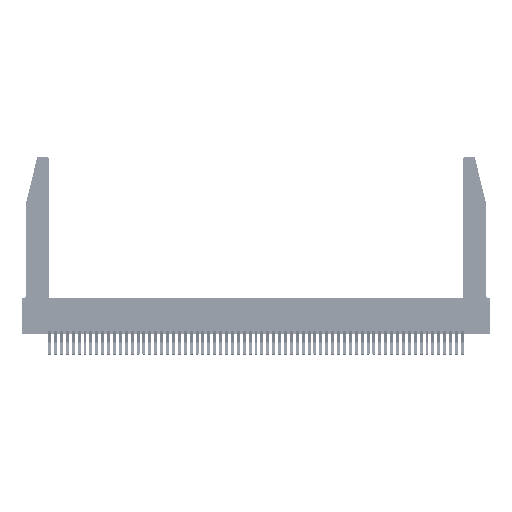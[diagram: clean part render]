
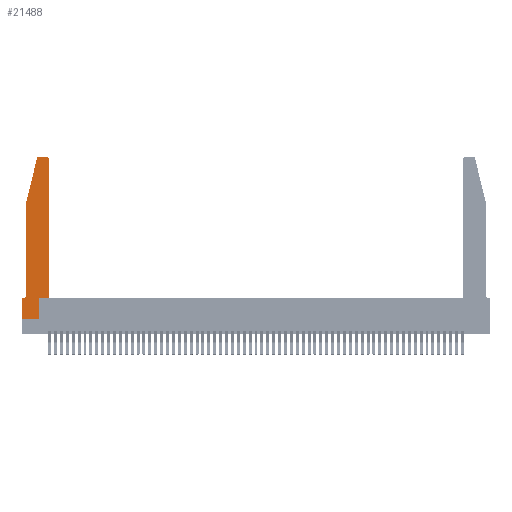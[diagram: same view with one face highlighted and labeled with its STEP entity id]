
A CAD part, top view. The second image highlights one B-rep face of the part: STEP entity #21488.
In plain terms, the highlighted planar face has unit normal (0, 0, 1).
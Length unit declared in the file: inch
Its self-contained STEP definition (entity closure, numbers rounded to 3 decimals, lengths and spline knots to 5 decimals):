
#803 = CARTESIAN_POINT ( 'NONE',  ( 0.0755, 2., 0.37 ) ) ;
#804 = EDGE_CURVE ( 'NONE', #41750, #5095, #30025, .T. ) ;
#1301 = CARTESIAN_POINT ( 'NONE',  ( 0.2865, 0., 0.37 ) ) ;
#1387 = CARTESIAN_POINT ( 'NONE',  ( 0.0055, 0.42, 0.37 ) ) ;
#2762 = VECTOR ( 'NONE', #8914, 39.37008 ) ;
#2973 = VECTOR ( 'NONE', #46245, 39.37008 ) ;
#4022 = EDGE_CURVE ( 'NONE', #11858, #41750, #15976, .T. ) ;
#4548 = VECTOR ( 'NONE', #15993, 39.37008 ) ;
#4670 = CARTESIAN_POINT ( 'NONE',  ( 0.4505, 0.35, 0.37 ) ) ;
#5095 = VERTEX_POINT ( 'NONE', #20547 ) ;
#5931 = DIRECTION ( 'NONE',  ( -1., 0., 0. ) ) ;
#6872 = VERTEX_POINT ( 'NONE', #18686 ) ;
#7213 = AXIS2_PLACEMENT_3D ( 'NONE', #19951, #37444, #11291 ) ;
#8715 = EDGE_LOOP ( 'NONE', ( #17613, #49337, #32407, #40443, #55276, #13586, #16196, #44043, #39970, #46020, #36558, #36023 ) ) ;
#8914 = DIRECTION ( 'NONE',  ( 0., -1., 0. ) ) ;
#9158 = DIRECTION ( 'NONE',  ( 1., 0., 0. ) ) ;
#9674 = LINE ( 'NONE', #45506, #54585 ) ;
#10699 = VERTEX_POINT ( 'NONE', #1301 ) ;
#11068 = VERTEX_POINT ( 'NONE', #38707 ) ;
#11097 = CIRCLE ( 'NONE', #44662, 0.03 ) ;
#11291 = DIRECTION ( 'NONE',  ( 1., 0., 0. ) ) ;
#11606 = EDGE_CURVE ( 'NONE', #55466, #10699, #17693, .T. ) ;
#11858 = VERTEX_POINT ( 'NONE', #48084 ) ;
#13586 = ORIENTED_EDGE ( 'NONE', *, *, #37803, .T. ) ;
#15199 = VECTOR ( 'NONE', #48949, 39.37008 ) ;
#15976 = LINE ( 'NONE', #48135, #2762 ) ;
#15993 = DIRECTION ( 'NONE',  ( 1., 0., 0. ) ) ;
#16196 = ORIENTED_EDGE ( 'NONE', *, *, #45359, .T. ) ;
#16296 = EDGE_CURVE ( 'NONE', #11068, #45266, #41244, .T. ) ;
#16573 = LINE ( 'NONE', #44597, #15199 ) ;
#16674 = CARTESIAN_POINT ( 'NONE',  ( 0.284, 2.72, 0.37 ) ) ;
#16882 = EDGE_CURVE ( 'NONE', #45266, #42300, #21484, .T. ) ;
#17613 = ORIENTED_EDGE ( 'NONE', *, *, #40620, .T. ) ;
#17693 = LINE ( 'NONE', #37718, #4548 ) ;
#17854 = VERTEX_POINT ( 'NONE', #32151 ) ;
#18579 = DIRECTION ( 'NONE',  ( 0., 0., 1. ) ) ;
#18686 = CARTESIAN_POINT ( 'NONE',  ( 0.284, 2.75, 0.37 ) ) ;
#19951 = CARTESIAN_POINT ( 'NONE',  ( 0., 0.35, 0.37 ) ) ;
#20547 = CARTESIAN_POINT ( 'NONE',  ( 0.0055, 0.35, 0.37 ) ) ;
#21099 = DIRECTION ( 'NONE',  ( 1., 0., 0. ) ) ;
#21484 = LINE ( 'NONE', #26206, #54690 ) ;
#21488 = ADVANCED_FACE ( 'NONE', ( #25038 ), #33116, .T. ) ;
#21638 = EDGE_CURVE ( 'NONE', #6872, #38180, #51411, .T. ) ;
#23947 = DIRECTION ( 'NONE',  ( -1., 0., 0. ) ) ;
#24023 = AXIS2_PLACEMENT_3D ( 'NONE', #1387, #32205, #5931 ) ;
#25038 = FACE_OUTER_BOUND ( 'NONE', #8715, .T. ) ;
#26206 = CARTESIAN_POINT ( 'NONE',  ( 0.4505, 0.35, 0.37 ) ) ;
#26783 = EDGE_CURVE ( 'NONE', #42300, #32089, #11097, .T. ) ;
#27752 = CARTESIAN_POINT ( 'NONE',  ( 0.4505, 2.72, 0.37 ) ) ;
#30025 = CIRCLE ( 'NONE', #24023, 0.07 ) ;
#30193 = CARTESIAN_POINT ( 'NONE',  ( 0.4505, 0.35, 0.37 ) ) ;
#30528 = DIRECTION ( 'NONE',  ( 0., 1., 0. ) ) ;
#30736 = AXIS2_PLACEMENT_3D ( 'NONE', #16674, #47074, #21099 ) ;
#31687 = DIRECTION ( 'NONE',  ( -0.239, -0.971, 0. ) ) ;
#32089 = VERTEX_POINT ( 'NONE', #39463 ) ;
#32151 = CARTESIAN_POINT ( 'NONE',  ( 0., 0.35, 0.37 ) ) ;
#32205 = DIRECTION ( 'NONE',  ( 0., 0., -1. ) ) ;
#32407 = ORIENTED_EDGE ( 'NONE', *, *, #42844, .T. ) ;
#33116 = PLANE ( 'NONE',  #7213 ) ;
#33411 = CARTESIAN_POINT ( 'NONE',  ( 0.2605, 2.75, 0.37 ) ) ;
#35023 = LINE ( 'NONE', #803, #45172 ) ;
#35095 = CARTESIAN_POINT ( 'NONE',  ( 0.25487, 2.72718, 0.37 ) ) ;
#36023 = ORIENTED_EDGE ( 'NONE', *, *, #26783, .T. ) ;
#36558 = ORIENTED_EDGE ( 'NONE', *, *, #16882, .T. ) ;
#36648 = LINE ( 'NONE', #33411, #2973 ) ;
#37444 = DIRECTION ( 'NONE',  ( 0., 0., 1. ) ) ;
#37659 = EDGE_CURVE ( 'NONE', #10699, #11068, #16573, .T. ) ;
#37718 = CARTESIAN_POINT ( 'NONE',  ( 0., 0., 0.37 ) ) ;
#37803 = EDGE_CURVE ( 'NONE', #5095, #17854, #9674, .T. ) ;
#38180 = VERTEX_POINT ( 'NONE', #35095 ) ;
#38308 = CARTESIAN_POINT ( 'NONE',  ( 0., 0., 0.37 ) ) ;
#38707 = CARTESIAN_POINT ( 'NONE',  ( 0.2865, 0.35, 0.37 ) ) ;
#39460 = CARTESIAN_POINT ( 'NONE',  ( 0., 0., 0.37 ) ) ;
#39463 = CARTESIAN_POINT ( 'NONE',  ( 0.4205, 2.75, 0.37 ) ) ;
#39970 = ORIENTED_EDGE ( 'NONE', *, *, #37659, .T. ) ;
#40443 = ORIENTED_EDGE ( 'NONE', *, *, #4022, .T. ) ;
#40620 = EDGE_CURVE ( 'NONE', #32089, #6872, #36648, .T. ) ;
#41244 = LINE ( 'NONE', #4670, #50037 ) ;
#41600 = VECTOR ( 'NONE', #52489, 39.37008 ) ;
#41750 = VERTEX_POINT ( 'NONE', #50100 ) ;
#42300 = VERTEX_POINT ( 'NONE', #27752 ) ;
#42844 = EDGE_CURVE ( 'NONE', #38180, #11858, #35023, .T. ) ;
#44043 = ORIENTED_EDGE ( 'NONE', *, *, #11606, .T. ) ;
#44597 = CARTESIAN_POINT ( 'NONE',  ( 0.2865, 0.35, 0.37 ) ) ;
#44631 = CARTESIAN_POINT ( 'NONE',  ( 0.4205, 2.72, 0.37 ) ) ;
#44662 = AXIS2_PLACEMENT_3D ( 'NONE', #44631, #18579, #48980 ) ;
#45172 = VECTOR ( 'NONE', #31687, 39.37008 ) ;
#45266 = VERTEX_POINT ( 'NONE', #30193 ) ;
#45359 = EDGE_CURVE ( 'NONE', #17854, #55466, #54442, .T. ) ;
#45506 = CARTESIAN_POINT ( 'NONE',  ( 0.0755, 0.35, 0.37 ) ) ;
#46020 = ORIENTED_EDGE ( 'NONE', *, *, #16296, .T. ) ;
#46245 = DIRECTION ( 'NONE',  ( -1., 0., 0. ) ) ;
#47074 = DIRECTION ( 'NONE',  ( 0., 0., 1. ) ) ;
#48084 = CARTESIAN_POINT ( 'NONE',  ( 0.0755, 2., 0.37 ) ) ;
#48135 = CARTESIAN_POINT ( 'NONE',  ( 0.0755, 2., 0.37 ) ) ;
#48949 = DIRECTION ( 'NONE',  ( 0., 1., 0. ) ) ;
#48980 = DIRECTION ( 'NONE',  ( 1., 0., 0. ) ) ;
#49337 = ORIENTED_EDGE ( 'NONE', *, *, #21638, .T. ) ;
#50037 = VECTOR ( 'NONE', #9158, 39.37008 ) ;
#50100 = CARTESIAN_POINT ( 'NONE',  ( 0.0755, 0.42, 0.37 ) ) ;
#51411 = CIRCLE ( 'NONE', #30736, 0.03 ) ;
#52489 = DIRECTION ( 'NONE',  ( 0., -1., 0. ) ) ;
#54442 = LINE ( 'NONE', #39460, #41600 ) ;
#54585 = VECTOR ( 'NONE', #23947, 39.37008 ) ;
#54690 = VECTOR ( 'NONE', #30528, 39.37008 ) ;
#55276 = ORIENTED_EDGE ( 'NONE', *, *, #804, .T. ) ;
#55466 = VERTEX_POINT ( 'NONE', #38308 ) ;
